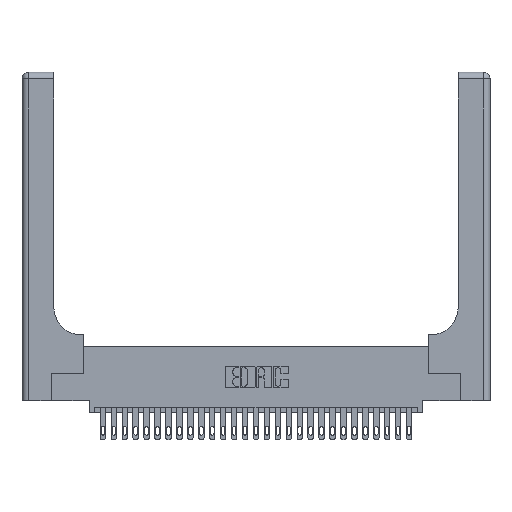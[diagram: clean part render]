
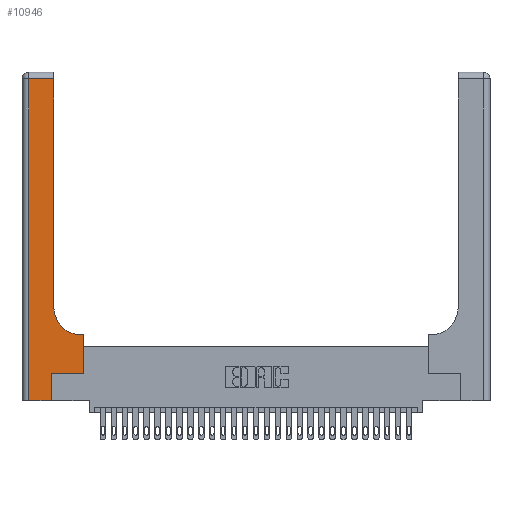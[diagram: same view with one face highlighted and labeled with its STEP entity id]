
A CAD part, top view. The second image highlights one B-rep face of the part: STEP entity #10946.
In plain terms, the highlighted planar face has unit normal (0, 0, 1).
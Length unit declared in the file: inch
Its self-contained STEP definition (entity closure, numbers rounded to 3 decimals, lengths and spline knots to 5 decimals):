
#943 = CARTESIAN_POINT ( 'NONE',  ( 0.2915, 0.6, 0.37 ) ) ;
#952 = EDGE_CURVE ( 'NONE', #24990, #13570, #25237, .T. ) ;
#965 = VECTOR ( 'NONE', #9110, 39.37008 ) ;
#1325 = CARTESIAN_POINT ( 'NONE',  ( 0., 2.94, 0.37 ) ) ;
#1401 = FACE_OUTER_BOUND ( 'NONE', #23526, .T. ) ;
#1645 = VERTEX_POINT ( 'NONE', #11807 ) ;
#2245 = LINE ( 'NONE', #25493, #20210 ) ;
#2556 = LINE ( 'NONE', #943, #24116 ) ;
#2895 = ORIENTED_EDGE ( 'NONE', *, *, #14408, .T. ) ;
#3201 = PLANE ( 'NONE',  #7924 ) ;
#3508 = AXIS2_PLACEMENT_3D ( 'NONE', #5548, #26615, #10171 ) ;
#3814 = CARTESIAN_POINT ( 'NONE',  ( 0.5585, 0.6, 0.37 ) ) ;
#4474 = CARTESIAN_POINT ( 'NONE',  ( 0.269, 0.25, 0.37 ) ) ;
#5414 = DIRECTION ( 'NONE',  ( 0., 1., 0. ) ) ;
#5498 = VERTEX_POINT ( 'NONE', #5518 ) ;
#5518 = CARTESIAN_POINT ( 'NONE',  ( 0.269, 0., 0.37 ) ) ;
#5548 = CARTESIAN_POINT ( 'NONE',  ( 0.5415, 0.85, 0.37 ) ) ;
#5785 = VECTOR ( 'NONE', #12608, 39.37008 ) ;
#6218 = CARTESIAN_POINT ( 'NONE',  ( 0., 0., 0.37 ) ) ;
#6407 = VECTOR ( 'NONE', #28380, 39.37008 ) ;
#6646 = ORIENTED_EDGE ( 'NONE', *, *, #13150, .T. ) ;
#7066 = LINE ( 'NONE', #1325, #19986 ) ;
#7116 = LINE ( 'NONE', #4474, #965 ) ;
#7236 = ORIENTED_EDGE ( 'NONE', *, *, #29559, .T. ) ;
#7700 = ORIENTED_EDGE ( 'NONE', *, *, #13500, .T. ) ;
#7906 = ORIENTED_EDGE ( 'NONE', *, *, #952, .T. ) ;
#7924 = AXIS2_PLACEMENT_3D ( 'NONE', #8676, #13278, #14428 ) ;
#8676 = CARTESIAN_POINT ( 'NONE',  ( 0., 3., 0.37 ) ) ;
#9110 = DIRECTION ( 'NONE',  ( 1., 0., 0. ) ) ;
#9272 = CIRCLE ( 'NONE', #3508, 0.25 ) ;
#10171 = DIRECTION ( 'NONE',  ( 1., 0., 0. ) ) ;
#10561 = EDGE_CURVE ( 'NONE', #13570, #5498, #17255, .T. ) ;
#10630 = CARTESIAN_POINT ( 'NONE',  ( 0.269, 0.25, 0.37 ) ) ;
#10758 = LINE ( 'NONE', #18827, #19712 ) ;
#10946 = ADVANCED_FACE ( 'NONE', ( #1401 ), #3201, .F. ) ;
#11807 = CARTESIAN_POINT ( 'NONE',  ( 0.2915, 2.94, 0.37 ) ) ;
#12267 = DIRECTION ( 'NONE',  ( -1., 0., 0. ) ) ;
#12608 = DIRECTION ( 'NONE',  ( 1., 0., 0. ) ) ;
#12628 = ORIENTED_EDGE ( 'NONE', *, *, #22339, .T. ) ;
#12662 = CARTESIAN_POINT ( 'NONE',  ( 0.5585, 0.25, 0.37 ) ) ;
#13150 = EDGE_CURVE ( 'NONE', #24859, #21724, #9272, .T. ) ;
#13278 = DIRECTION ( 'NONE',  ( 0., 0., -1. ) ) ;
#13500 = EDGE_CURVE ( 'NONE', #1645, #24990, #7066, .T. ) ;
#13570 = VERTEX_POINT ( 'NONE', #23811 ) ;
#14408 = EDGE_CURVE ( 'NONE', #16296, #26785, #26503, .T. ) ;
#14428 = DIRECTION ( 'NONE',  ( -1., 0., 0. ) ) ;
#14455 = VECTOR ( 'NONE', #14712, 39.37008 ) ;
#14712 = DIRECTION ( 'NONE',  ( 0., -1., 0. ) ) ;
#14878 = EDGE_CURVE ( 'NONE', #27879, #16296, #7116, .T. ) ;
#16296 = VERTEX_POINT ( 'NONE', #12662 ) ;
#16345 = DIRECTION ( 'NONE',  ( 0., 1., 0. ) ) ;
#16782 = DIRECTION ( 'NONE',  ( -1., 0., 0. ) ) ;
#17255 = LINE ( 'NONE', #6218, #5785 ) ;
#17924 = EDGE_CURVE ( 'NONE', #5498, #27879, #2245, .T. ) ;
#18827 = CARTESIAN_POINT ( 'NONE',  ( 0.2915, 3., 0.37 ) ) ;
#19290 = CARTESIAN_POINT ( 'NONE',  ( 0.06, 3., 0.37 ) ) ;
#19460 = CARTESIAN_POINT ( 'NONE',  ( 0.2915, 0.85, 0.37 ) ) ;
#19712 = VECTOR ( 'NONE', #5414, 39.37008 ) ;
#19755 = ORIENTED_EDGE ( 'NONE', *, *, #17924, .T. ) ;
#19986 = VECTOR ( 'NONE', #16782, 39.37008 ) ;
#20210 = VECTOR ( 'NONE', #16345, 39.37008 ) ;
#21084 = CARTESIAN_POINT ( 'NONE',  ( 0.5415, 0.6, 0.37 ) ) ;
#21724 = VERTEX_POINT ( 'NONE', #19460 ) ;
#22339 = EDGE_CURVE ( 'NONE', #21724, #1645, #10758, .T. ) ;
#23526 = EDGE_LOOP ( 'NONE', ( #12628, #7700, #7906, #23608, #19755, #28233, #2895, #7236, #6646 ) ) ;
#23608 = ORIENTED_EDGE ( 'NONE', *, *, #10561, .T. ) ;
#23778 = CARTESIAN_POINT ( 'NONE',  ( 0.5585, 0.25, 0.37 ) ) ;
#23811 = CARTESIAN_POINT ( 'NONE',  ( 0.06, 0., 0.37 ) ) ;
#24003 = CARTESIAN_POINT ( 'NONE',  ( 0.06, 2.94, 0.37 ) ) ;
#24116 = VECTOR ( 'NONE', #12267, 39.37008 ) ;
#24859 = VERTEX_POINT ( 'NONE', #21084 ) ;
#24990 = VERTEX_POINT ( 'NONE', #24003 ) ;
#25237 = LINE ( 'NONE', #19290, #14455 ) ;
#25493 = CARTESIAN_POINT ( 'NONE',  ( 0.269, 0., 0.37 ) ) ;
#26503 = LINE ( 'NONE', #23778, #6407 ) ;
#26615 = DIRECTION ( 'NONE',  ( 0., 0., -1. ) ) ;
#26785 = VERTEX_POINT ( 'NONE', #3814 ) ;
#27879 = VERTEX_POINT ( 'NONE', #10630 ) ;
#28233 = ORIENTED_EDGE ( 'NONE', *, *, #14878, .T. ) ;
#28380 = DIRECTION ( 'NONE',  ( 0., 1., 0. ) ) ;
#29559 = EDGE_CURVE ( 'NONE', #26785, #24859, #2556, .T. ) ;
